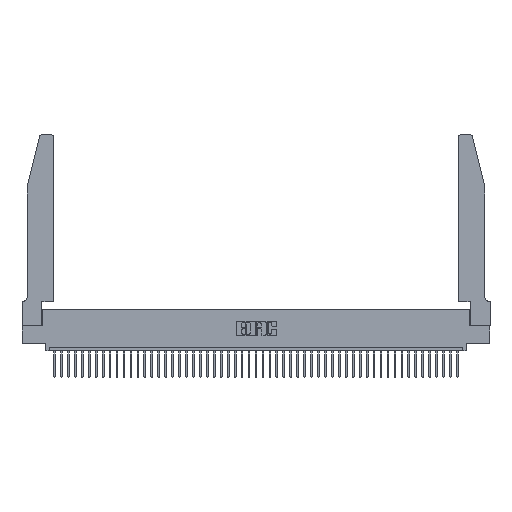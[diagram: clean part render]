
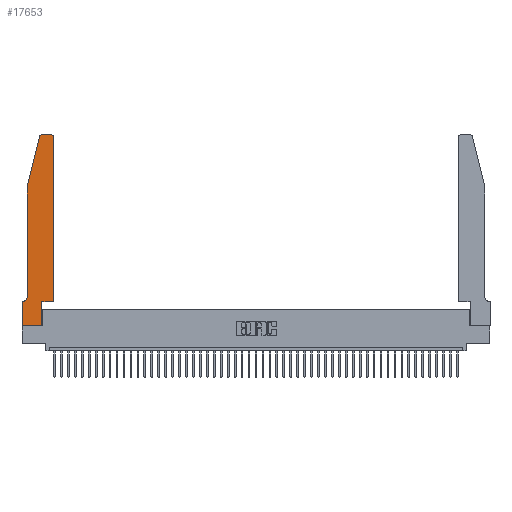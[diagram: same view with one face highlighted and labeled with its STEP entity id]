
A CAD part, top view. The second image highlights one B-rep face of the part: STEP entity #17653.
In plain terms, the highlighted planar face has unit normal (0, 0, 1).
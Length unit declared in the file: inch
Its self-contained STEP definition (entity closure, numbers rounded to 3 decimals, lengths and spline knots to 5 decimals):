
#640 = EDGE_CURVE ( 'NONE', #23289, #44212, #25825, .T. ) ;
#685 = LINE ( 'NONE', #17534, #17942 ) ;
#2389 = EDGE_CURVE ( 'NONE', #11214, #12948, #36792, .T. ) ;
#2905 = CARTESIAN_POINT ( 'NONE',  ( 0.4205, 2.75, 0.37 ) ) ;
#3142 = DIRECTION ( 'NONE',  ( -1., 0., 0. ) ) ;
#4460 = CIRCLE ( 'NONE', #40583, 0.03 ) ;
#4504 = DIRECTION ( 'NONE',  ( 0., -1., 0. ) ) ;
#6521 = EDGE_CURVE ( 'NONE', #24710, #34973, #4460, .T. ) ;
#6598 = DIRECTION ( 'NONE',  ( 0., 0., -1. ) ) ;
#6851 = ORIENTED_EDGE ( 'NONE', *, *, #28316, .T. ) ;
#7144 = EDGE_CURVE ( 'NONE', #34973, #23289, #35014, .T. ) ;
#7154 = DIRECTION ( 'NONE',  ( 0., 1., 0. ) ) ;
#7591 = VERTEX_POINT ( 'NONE', #44457 ) ;
#8098 = EDGE_CURVE ( 'NONE', #18376, #21246, #26495, .T. ) ;
#8527 = CARTESIAN_POINT ( 'NONE',  ( 0.4505, 0.35, 0.37 ) ) ;
#8734 = EDGE_CURVE ( 'NONE', #44212, #41593, #42994, .T. ) ;
#11214 = VERTEX_POINT ( 'NONE', #18082 ) ;
#12444 = CARTESIAN_POINT ( 'NONE',  ( 0., 0.35, 0.37 ) ) ;
#12948 = VERTEX_POINT ( 'NONE', #8527 ) ;
#13156 = VECTOR ( 'NONE', #44483, 39.37008 ) ;
#13435 = LINE ( 'NONE', #28293, #40081 ) ;
#13707 = VECTOR ( 'NONE', #17843, 39.37008 ) ;
#14170 = CARTESIAN_POINT ( 'NONE',  ( 0.2865, 0.35, 0.37 ) ) ;
#14185 = CARTESIAN_POINT ( 'NONE',  ( 0.25487, 2.72718, 0.37 ) ) ;
#14209 = ORIENTED_EDGE ( 'NONE', *, *, #33478, .T. ) ;
#17534 = CARTESIAN_POINT ( 'NONE',  ( 0.0755, 0.35, 0.37 ) ) ;
#17587 = PLANE ( 'NONE',  #45131 ) ;
#17653 = ADVANCED_FACE ( 'NONE', ( #17720 ), #17587, .T. ) ;
#17720 = FACE_OUTER_BOUND ( 'NONE', #44689, .T. ) ;
#17777 = CARTESIAN_POINT ( 'NONE',  ( 0.0055, 0.42, 0.37 ) ) ;
#17843 = DIRECTION ( 'NONE',  ( 0., 1., 0. ) ) ;
#17942 = VECTOR ( 'NONE', #3142, 39.37008 ) ;
#18082 = CARTESIAN_POINT ( 'NONE',  ( 0.2865, 0.35, 0.37 ) ) ;
#18376 = VERTEX_POINT ( 'NONE', #22436 ) ;
#19078 = LINE ( 'NONE', #25873, #45799 ) ;
#19898 = ORIENTED_EDGE ( 'NONE', *, *, #32543, .T. ) ;
#20238 = ORIENTED_EDGE ( 'NONE', *, *, #640, .T. ) ;
#21246 = VERTEX_POINT ( 'NONE', #2905 ) ;
#21652 = CARTESIAN_POINT ( 'NONE',  ( 0.4505, 0.35, 0.37 ) ) ;
#21697 = DIRECTION ( 'NONE',  ( 1., 0., 0. ) ) ;
#21938 = VECTOR ( 'NONE', #37169, 39.37008 ) ;
#22190 = DIRECTION ( 'NONE',  ( 1., 0., 0. ) ) ;
#22436 = CARTESIAN_POINT ( 'NONE',  ( 0.4505, 2.72, 0.37 ) ) ;
#22551 = ORIENTED_EDGE ( 'NONE', *, *, #7144, .T. ) ;
#23289 = VERTEX_POINT ( 'NONE', #43443 ) ;
#23961 = ORIENTED_EDGE ( 'NONE', *, *, #27666, .T. ) ;
#24274 = CARTESIAN_POINT ( 'NONE',  ( 0.0755, 0.42, 0.37 ) ) ;
#24710 = VERTEX_POINT ( 'NONE', #31146 ) ;
#25418 = ORIENTED_EDGE ( 'NONE', *, *, #6521, .T. ) ;
#25825 = LINE ( 'NONE', #29025, #41093 ) ;
#25873 = CARTESIAN_POINT ( 'NONE',  ( 0., 0., 0.37 ) ) ;
#26231 = CARTESIAN_POINT ( 'NONE',  ( 0.0755, 2., 0.37 ) ) ;
#26495 = CIRCLE ( 'NONE', #40073, 0.03 ) ;
#26556 = LINE ( 'NONE', #21652, #33429 ) ;
#27666 = EDGE_CURVE ( 'NONE', #7591, #44813, #19078, .T. ) ;
#27714 = CARTESIAN_POINT ( 'NONE',  ( 0.4205, 2.72, 0.37 ) ) ;
#28293 = CARTESIAN_POINT ( 'NONE',  ( 0., 0., 0.37 ) ) ;
#28316 = EDGE_CURVE ( 'NONE', #30251, #7591, #13435, .T. ) ;
#28612 = EDGE_CURVE ( 'NONE', #41593, #30251, #685, .T. ) ;
#29025 = CARTESIAN_POINT ( 'NONE',  ( 0.0755, 2., 0.37 ) ) ;
#29724 = CARTESIAN_POINT ( 'NONE',  ( 0.2605, 2.75, 0.37 ) ) ;
#30251 = VERTEX_POINT ( 'NONE', #12444 ) ;
#31146 = CARTESIAN_POINT ( 'NONE',  ( 0.284, 2.75, 0.37 ) ) ;
#31366 = ORIENTED_EDGE ( 'NONE', *, *, #31581, .T. ) ;
#31581 = EDGE_CURVE ( 'NONE', #44813, #11214, #40340, .T. ) ;
#32149 = CARTESIAN_POINT ( 'NONE',  ( 0.2865, 0., 0.37 ) ) ;
#32433 = LINE ( 'NONE', #29724, #13156 ) ;
#32543 = EDGE_CURVE ( 'NONE', #21246, #24710, #32433, .T. ) ;
#33429 = VECTOR ( 'NONE', #7154, 39.37008 ) ;
#33478 = EDGE_CURVE ( 'NONE', #12948, #18376, #26556, .T. ) ;
#33597 = DIRECTION ( 'NONE',  ( 1., 0., 0. ) ) ;
#34552 = DIRECTION ( 'NONE',  ( 0., 0., 1. ) ) ;
#34973 = VERTEX_POINT ( 'NONE', #14185 ) ;
#35014 = LINE ( 'NONE', #26231, #21938 ) ;
#35978 = CARTESIAN_POINT ( 'NONE',  ( 0., 0.35, 0.37 ) ) ;
#36012 = ORIENTED_EDGE ( 'NONE', *, *, #28612, .T. ) ;
#36205 = DIRECTION ( 'NONE',  ( 0., 0., 1. ) ) ;
#36633 = CARTESIAN_POINT ( 'NONE',  ( 0.284, 2.72, 0.37 ) ) ;
#36792 = LINE ( 'NONE', #41196, #46989 ) ;
#37169 = DIRECTION ( 'NONE',  ( -0.239, -0.971, 0. ) ) ;
#37618 = ORIENTED_EDGE ( 'NONE', *, *, #2389, .T. ) ;
#37697 = DIRECTION ( 'NONE',  ( 1., 0., 0. ) ) ;
#38557 = CARTESIAN_POINT ( 'NONE',  ( 0.0055, 0.35, 0.37 ) ) ;
#39355 = DIRECTION ( 'NONE',  ( -1., 0., 0. ) ) ;
#39795 = DIRECTION ( 'NONE',  ( 0., 0., 1. ) ) ;
#40073 = AXIS2_PLACEMENT_3D ( 'NONE', #27714, #34552, #41705 ) ;
#40081 = VECTOR ( 'NONE', #4504, 39.37008 ) ;
#40340 = LINE ( 'NONE', #14170, #13707 ) ;
#40390 = ORIENTED_EDGE ( 'NONE', *, *, #8098, .T. ) ;
#40583 = AXIS2_PLACEMENT_3D ( 'NONE', #36633, #36205, #22190 ) ;
#41093 = VECTOR ( 'NONE', #46965, 39.37008 ) ;
#41196 = CARTESIAN_POINT ( 'NONE',  ( 0.4505, 0.35, 0.37 ) ) ;
#41593 = VERTEX_POINT ( 'NONE', #38557 ) ;
#41705 = DIRECTION ( 'NONE',  ( 1., 0., 0. ) ) ;
#42994 = CIRCLE ( 'NONE', #46434, 0.07 ) ;
#43443 = CARTESIAN_POINT ( 'NONE',  ( 0.0755, 2., 0.37 ) ) ;
#43618 = ORIENTED_EDGE ( 'NONE', *, *, #8734, .T. ) ;
#44212 = VERTEX_POINT ( 'NONE', #24274 ) ;
#44457 = CARTESIAN_POINT ( 'NONE',  ( 0., 0., 0.37 ) ) ;
#44483 = DIRECTION ( 'NONE',  ( -1., 0., 0. ) ) ;
#44689 = EDGE_LOOP ( 'NONE', ( #19898, #25418, #22551, #20238, #43618, #36012, #6851, #23961, #31366, #37618, #14209, #40390 ) ) ;
#44813 = VERTEX_POINT ( 'NONE', #32149 ) ;
#45131 = AXIS2_PLACEMENT_3D ( 'NONE', #35978, #39795, #21697 ) ;
#45799 = VECTOR ( 'NONE', #33597, 39.37008 ) ;
#46434 = AXIS2_PLACEMENT_3D ( 'NONE', #17777, #6598, #39355 ) ;
#46965 = DIRECTION ( 'NONE',  ( 0., -1., 0. ) ) ;
#46989 = VECTOR ( 'NONE', #37697, 39.37008 ) ;
